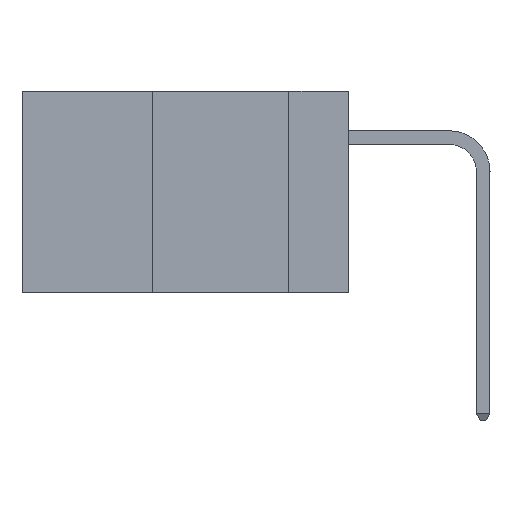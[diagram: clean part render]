
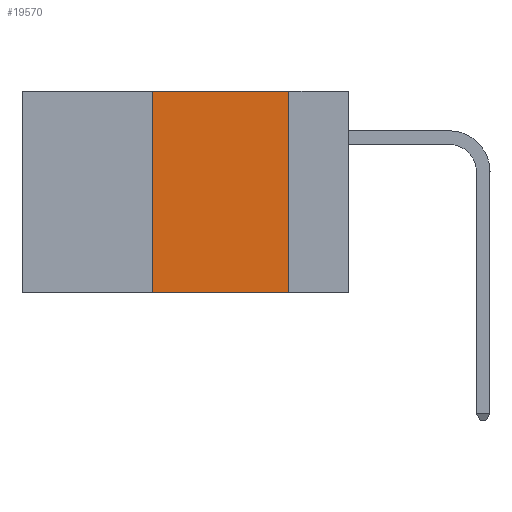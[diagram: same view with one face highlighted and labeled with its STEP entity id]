
A CAD part, left-side view. The second image highlights one B-rep face of the part: STEP entity #19570.
In plain terms, the highlighted planar face has unit normal (-1, 0, 0).
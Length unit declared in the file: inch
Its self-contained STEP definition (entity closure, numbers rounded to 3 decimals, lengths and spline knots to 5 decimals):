
#3578 = EDGE_CURVE ( 'NONE', #31246, #24356, #40381, .T. ) ;
#5727 = VERTEX_POINT ( 'NONE', #18593 ) ;
#5965 = EDGE_CURVE ( 'NONE', #24356, #35018, #31619, .T. ) ;
#7640 = VECTOR ( 'NONE', #22685, 39.37008 ) ;
#8544 = CARTESIAN_POINT ( 'NONE',  ( 0., 0.36, 0. ) ) ;
#14136 = DIRECTION ( 'NONE',  ( 1., 0., 0. ) ) ;
#18593 = CARTESIAN_POINT ( 'NONE',  ( 0., 0.11, -0.37 ) ) ;
#18784 = CARTESIAN_POINT ( 'NONE',  ( 0., 0.11, 0. ) ) ;
#19570 = ADVANCED_FACE ( 'NONE', ( #28952 ), #37373, .F. ) ;
#20162 = ORIENTED_EDGE ( 'NONE', *, *, #36590, .F. ) ;
#20361 = AXIS2_PLACEMENT_3D ( 'NONE', #37212, #14136, #41267 ) ;
#22685 = DIRECTION ( 'NONE',  ( 0., 0., -1. ) ) ;
#24356 = VERTEX_POINT ( 'NONE', #34749 ) ;
#25400 = ORIENTED_EDGE ( 'NONE', *, *, #31691, .T. ) ;
#28632 = CARTESIAN_POINT ( 'NONE',  ( 0., 0.11, 0. ) ) ;
#28952 = FACE_OUTER_BOUND ( 'NONE', #34149, .T. ) ;
#29593 = LINE ( 'NONE', #18784, #7640 ) ;
#30039 = ORIENTED_EDGE ( 'NONE', *, *, #5965, .F. ) ;
#31246 = VERTEX_POINT ( 'NONE', #45185 ) ;
#31619 = LINE ( 'NONE', #47201, #40696 ) ;
#31691 = EDGE_CURVE ( 'NONE', #31246, #5727, #39195, .T. ) ;
#33995 = ORIENTED_EDGE ( 'NONE', *, *, #3578, .F. ) ;
#34149 = EDGE_LOOP ( 'NONE', ( #20162, #30039, #33995, #25400 ) ) ;
#34749 = CARTESIAN_POINT ( 'NONE',  ( 0., 0.36, 0. ) ) ;
#35018 = VERTEX_POINT ( 'NONE', #28632 ) ;
#36590 = EDGE_CURVE ( 'NONE', #35018, #5727, #29593, .T. ) ;
#37212 = CARTESIAN_POINT ( 'NONE',  ( 0., 0.6, 0. ) ) ;
#37373 = PLANE ( 'NONE',  #20361 ) ;
#39195 = LINE ( 'NONE', #43041, #48211 ) ;
#39644 = DIRECTION ( 'NONE',  ( 0., 0., 1. ) ) ;
#40381 = LINE ( 'NONE', #8544, #49358 ) ;
#40696 = VECTOR ( 'NONE', #43318, 39.37008 ) ;
#41267 = DIRECTION ( 'NONE',  ( 0., 0., -1. ) ) ;
#43041 = CARTESIAN_POINT ( 'NONE',  ( 0., 0.6, -0.37 ) ) ;
#43318 = DIRECTION ( 'NONE',  ( 0., -1., 0. ) ) ;
#45185 = CARTESIAN_POINT ( 'NONE',  ( 0., 0.36, -0.37 ) ) ;
#46920 = DIRECTION ( 'NONE',  ( 0., -1., 0. ) ) ;
#47201 = CARTESIAN_POINT ( 'NONE',  ( 0., 0.6, 0. ) ) ;
#48211 = VECTOR ( 'NONE', #46920, 39.37008 ) ;
#49358 = VECTOR ( 'NONE', #39644, 39.37008 ) ;
